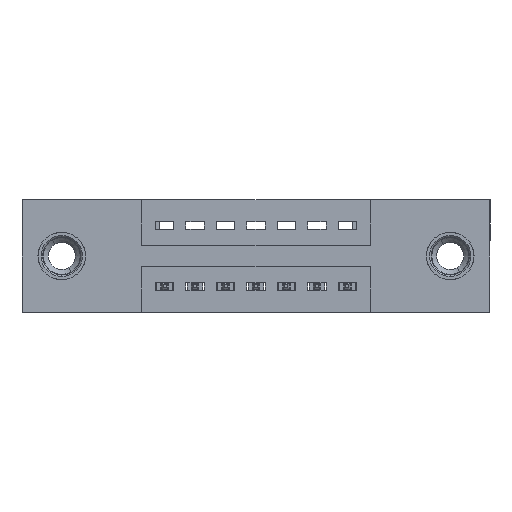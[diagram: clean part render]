
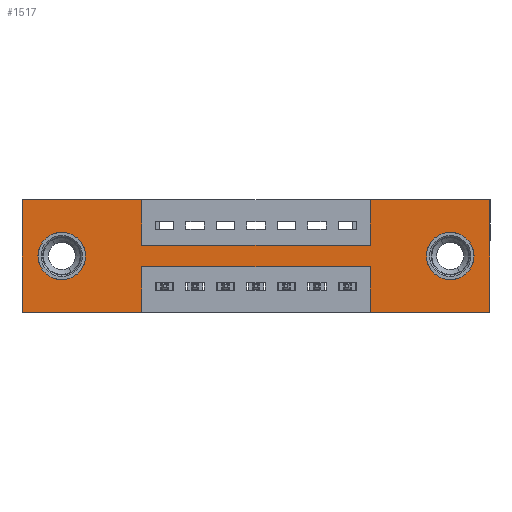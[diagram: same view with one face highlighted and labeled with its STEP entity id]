
A CAD part, front view. The second image highlights one B-rep face of the part: STEP entity #1517.
In plain terms, the highlighted planar face has unit normal (0, -1, 0).
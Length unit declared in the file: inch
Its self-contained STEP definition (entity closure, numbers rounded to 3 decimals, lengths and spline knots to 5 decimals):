
#113 = VERTEX_POINT ( 'NONE', #7295 ) ;
#277 = ORIENTED_EDGE ( 'NONE', *, *, #6809, .F. ) ;
#323 = VERTEX_POINT ( 'NONE', #5345 ) ;
#360 = CARTESIAN_POINT ( 'NONE',  ( 0.13, 0., -0.263 ) ) ;
#495 = EDGE_CURVE ( 'NONE', #4745, #14219, #9476, .T. ) ;
#669 = CARTESIAN_POINT ( 'NONE',  ( 1.405, 0., -0.185 ) ) ;
#693 = EDGE_CURVE ( 'NONE', #113, #14028, #1950, .T. ) ;
#728 = AXIS2_PLACEMENT_3D ( 'NONE', #6115, #1518, #10643 ) ;
#738 = ORIENTED_EDGE ( 'NONE', *, *, #2934, .F. ) ;
#791 = LINE ( 'NONE', #8367, #1706 ) ;
#948 = CARTESIAN_POINT ( 'NONE',  ( 1.535, 0., 0. ) ) ;
#960 = EDGE_CURVE ( 'NONE', #10817, #13637, #3906, .T. ) ;
#1022 = CARTESIAN_POINT ( 'NONE',  ( 0., 0., 0. ) ) ;
#1066 = CARTESIAN_POINT ( 'NONE',  ( 0.3925, 0., -0.37 ) ) ;
#1148 = DIRECTION ( 'NONE',  ( -1., 0., 0. ) ) ;
#1242 = ORIENTED_EDGE ( 'NONE', *, *, #4213, .F. ) ;
#1282 = AXIS2_PLACEMENT_3D ( 'NONE', #13565, #6637, #8975 ) ;
#1306 = ORIENTED_EDGE ( 'NONE', *, *, #960, .T. ) ;
#1517 = ADVANCED_FACE ( 'NONE', ( #7096, #2469, #4066 ), #3292, .T. ) ;
#1518 = DIRECTION ( 'NONE',  ( 0., 1., 0. ) ) ;
#1637 = ORIENTED_EDGE ( 'NONE', *, *, #8611, .F. ) ;
#1706 = VECTOR ( 'NONE', #1148, 39.37008 ) ;
#1950 = LINE ( 'NONE', #1022, #2303 ) ;
#1959 = CARTESIAN_POINT ( 'NONE',  ( 1.1425, 0., 0. ) ) ;
#1962 = CARTESIAN_POINT ( 'NONE',  ( 1.1425, 0., -0.15 ) ) ;
#2038 = AXIS2_PLACEMENT_3D ( 'NONE', #669, #14268, #8656 ) ;
#2050 = DIRECTION ( 'NONE',  ( 0., 0., 1. ) ) ;
#2103 = AXIS2_PLACEMENT_3D ( 'NONE', #7511, #5322, #13303 ) ;
#2284 = CARTESIAN_POINT ( 'NONE',  ( 0.3925, 0., 0. ) ) ;
#2303 = VECTOR ( 'NONE', #2050, 39.37008 ) ;
#2421 = VERTEX_POINT ( 'NONE', #4828 ) ;
#2469 = FACE_BOUND ( 'NONE', #14363, .T. ) ;
#2500 = ORIENTED_EDGE ( 'NONE', *, *, #9131, .F. ) ;
#2554 = DIRECTION ( 'NONE',  ( 0., 1., 0. ) ) ;
#2634 = CARTESIAN_POINT ( 'NONE',  ( 0.3925, 0., -0.22 ) ) ;
#2934 = EDGE_CURVE ( 'NONE', #9582, #8300, #12788, .T. ) ;
#2944 = LINE ( 'NONE', #948, #11658 ) ;
#3166 = DIRECTION ( 'NONE',  ( 0., 0., -1. ) ) ;
#3292 = PLANE ( 'NONE',  #1282 ) ;
#3645 = ORIENTED_EDGE ( 'NONE', *, *, #4347, .F. ) ;
#3849 = ORIENTED_EDGE ( 'NONE', *, *, #4507, .T. ) ;
#3906 = CIRCLE ( 'NONE', #8739, 0.078 ) ;
#4066 = FACE_OUTER_BOUND ( 'NONE', #9863, .T. ) ;
#4147 = DIRECTION ( 'NONE',  ( -1., 0., 0. ) ) ;
#4213 = EDGE_CURVE ( 'NONE', #11469, #14191, #9954, .T. ) ;
#4347 = EDGE_CURVE ( 'NONE', #14191, #113, #791, .T. ) ;
#4355 = ORIENTED_EDGE ( 'NONE', *, *, #5739, .F. ) ;
#4430 = CARTESIAN_POINT ( 'NONE',  ( 0., 0., 0. ) ) ;
#4507 = EDGE_CURVE ( 'NONE', #13637, #10817, #5997, .T. ) ;
#4537 = LINE ( 'NONE', #5249, #12949 ) ;
#4667 = ORIENTED_EDGE ( 'NONE', *, *, #693, .F. ) ;
#4745 = VERTEX_POINT ( 'NONE', #1959 ) ;
#4828 = CARTESIAN_POINT ( 'NONE',  ( 1.535, 0., -0.37 ) ) ;
#4985 = DIRECTION ( 'NONE',  ( 0., 0., 1. ) ) ;
#5249 = CARTESIAN_POINT ( 'NONE',  ( 0., 0., -0.37 ) ) ;
#5322 = DIRECTION ( 'NONE',  ( 0., 1., 0. ) ) ;
#5345 = CARTESIAN_POINT ( 'NONE',  ( 1.405, 0., -0.263 ) ) ;
#5379 = EDGE_CURVE ( 'NONE', #14385, #323, #12201, .T. ) ;
#5446 = EDGE_LOOP ( 'NONE', ( #7720, #6292 ) ) ;
#5739 = EDGE_CURVE ( 'NONE', #14219, #2421, #2944, .T. ) ;
#5985 = CARTESIAN_POINT ( 'NONE',  ( 1.405, 0., -0.107 ) ) ;
#5997 = CIRCLE ( 'NONE', #728, 0.078 ) ;
#6115 = CARTESIAN_POINT ( 'NONE',  ( 0.13, 0., -0.185 ) ) ;
#6256 = CARTESIAN_POINT ( 'NONE',  ( 1.1425, 0., -0.37 ) ) ;
#6292 = ORIENTED_EDGE ( 'NONE', *, *, #9628, .T. ) ;
#6389 = CIRCLE ( 'NONE', #2038, 0.078 ) ;
#6414 = DIRECTION ( 'NONE',  ( -1., 0., 0. ) ) ;
#6459 = EDGE_CURVE ( 'NONE', #14028, #9582, #10750, .T. ) ;
#6483 = VERTEX_POINT ( 'NONE', #7733 ) ;
#6513 = VERTEX_POINT ( 'NONE', #1962 ) ;
#6637 = DIRECTION ( 'NONE',  ( 0., -1., 0. ) ) ;
#6786 = VERTEX_POINT ( 'NONE', #8350 ) ;
#6809 = EDGE_CURVE ( 'NONE', #6513, #4745, #8425, .T. ) ;
#7096 = FACE_BOUND ( 'NONE', #5446, .T. ) ;
#7295 = CARTESIAN_POINT ( 'NONE',  ( 0., 0., -0.37 ) ) ;
#7365 = CARTESIAN_POINT ( 'NONE',  ( 0.3925, 0., 0. ) ) ;
#7488 = ORIENTED_EDGE ( 'NONE', *, *, #6459, .F. ) ;
#7511 = CARTESIAN_POINT ( 'NONE',  ( 1.405, 0., -0.185 ) ) ;
#7706 = VECTOR ( 'NONE', #11027, 39.37008 ) ;
#7720 = ORIENTED_EDGE ( 'NONE', *, *, #5379, .T. ) ;
#7733 = CARTESIAN_POINT ( 'NONE',  ( 1.1425, 0., -0.37 ) ) ;
#7863 = CARTESIAN_POINT ( 'NONE',  ( 0.3925, 0., -0.15 ) ) ;
#7884 = DIRECTION ( 'NONE',  ( 0., 0., -1. ) ) ;
#8300 = VERTEX_POINT ( 'NONE', #10331 ) ;
#8350 = CARTESIAN_POINT ( 'NONE',  ( 1.1425, 0., -0.22 ) ) ;
#8367 = CARTESIAN_POINT ( 'NONE',  ( 0., 0., -0.37 ) ) ;
#8425 = LINE ( 'NONE', #10886, #9696 ) ;
#8579 = DIRECTION ( 'NONE',  ( 0., 0., 1. ) ) ;
#8611 = EDGE_CURVE ( 'NONE', #8300, #6513, #11574, .T. ) ;
#8656 = DIRECTION ( 'NONE',  ( 0., 0., -1. ) ) ;
#8739 = AXIS2_PLACEMENT_3D ( 'NONE', #10676, #2554, #4985 ) ;
#8975 = DIRECTION ( 'NONE',  ( 0., 0., -1. ) ) ;
#9131 = EDGE_CURVE ( 'NONE', #6786, #11469, #10685, .T. ) ;
#9382 = VECTOR ( 'NONE', #8579, 39.37008 ) ;
#9476 = LINE ( 'NONE', #4430, #13935 ) ;
#9582 = VERTEX_POINT ( 'NONE', #7365 ) ;
#9628 = EDGE_CURVE ( 'NONE', #323, #14385, #6389, .T. ) ;
#9696 = VECTOR ( 'NONE', #14321, 39.37008 ) ;
#9863 = EDGE_LOOP ( 'NONE', ( #1242, #2500, #14720, #12967, #4355, #14806, #277, #1637, #738, #7488, #4667, #3645 ) ) ;
#9954 = LINE ( 'NONE', #12232, #11730 ) ;
#9975 = CARTESIAN_POINT ( 'NONE',  ( 0., 0., 0. ) ) ;
#10151 = VECTOR ( 'NONE', #6414, 39.37008 ) ;
#10331 = CARTESIAN_POINT ( 'NONE',  ( 0.3925, 0., -0.15 ) ) ;
#10643 = DIRECTION ( 'NONE',  ( 0., 0., 1. ) ) ;
#10676 = CARTESIAN_POINT ( 'NONE',  ( 0.13, 0., -0.185 ) ) ;
#10685 = LINE ( 'NONE', #12040, #10151 ) ;
#10750 = LINE ( 'NONE', #14410, #7706 ) ;
#10817 = VERTEX_POINT ( 'NONE', #360 ) ;
#10886 = CARTESIAN_POINT ( 'NONE',  ( 1.1425, 0., 0. ) ) ;
#11027 = DIRECTION ( 'NONE',  ( 1., 0., 0. ) ) ;
#11203 = DIRECTION ( 'NONE',  ( 1., 0., 0. ) ) ;
#11445 = DIRECTION ( 'NONE',  ( 0., 0., -1. ) ) ;
#11446 = CARTESIAN_POINT ( 'NONE',  ( 1.535, 0., 0. ) ) ;
#11469 = VERTEX_POINT ( 'NONE', #2634 ) ;
#11493 = LINE ( 'NONE', #6256, #9382 ) ;
#11533 = VECTOR ( 'NONE', #11445, 39.37008 ) ;
#11574 = LINE ( 'NONE', #7863, #14471 ) ;
#11658 = VECTOR ( 'NONE', #7884, 39.37008 ) ;
#11730 = VECTOR ( 'NONE', #3166, 39.37008 ) ;
#12040 = CARTESIAN_POINT ( 'NONE',  ( 0.3925, 0., -0.22 ) ) ;
#12201 = CIRCLE ( 'NONE', #2103, 0.078 ) ;
#12232 = CARTESIAN_POINT ( 'NONE',  ( 0.3925, 0., -0.37 ) ) ;
#12453 = DIRECTION ( 'NONE',  ( 1., 0., 0. ) ) ;
#12788 = LINE ( 'NONE', #2284, #11533 ) ;
#12949 = VECTOR ( 'NONE', #4147, 39.37008 ) ;
#12967 = ORIENTED_EDGE ( 'NONE', *, *, #13505, .F. ) ;
#13303 = DIRECTION ( 'NONE',  ( 0., 0., -1. ) ) ;
#13505 = EDGE_CURVE ( 'NONE', #2421, #6483, #4537, .T. ) ;
#13565 = CARTESIAN_POINT ( 'NONE',  ( 0., 0., -0.37 ) ) ;
#13637 = VERTEX_POINT ( 'NONE', #14686 ) ;
#13911 = EDGE_CURVE ( 'NONE', #6483, #6786, #11493, .T. ) ;
#13935 = VECTOR ( 'NONE', #11203, 39.37008 ) ;
#14028 = VERTEX_POINT ( 'NONE', #9975 ) ;
#14191 = VERTEX_POINT ( 'NONE', #1066 ) ;
#14219 = VERTEX_POINT ( 'NONE', #11446 ) ;
#14268 = DIRECTION ( 'NONE',  ( 0., 1., 0. ) ) ;
#14321 = DIRECTION ( 'NONE',  ( 0., 0., 1. ) ) ;
#14363 = EDGE_LOOP ( 'NONE', ( #3849, #1306 ) ) ;
#14385 = VERTEX_POINT ( 'NONE', #5985 ) ;
#14410 = CARTESIAN_POINT ( 'NONE',  ( 0., 0., 0. ) ) ;
#14471 = VECTOR ( 'NONE', #12453, 39.37008 ) ;
#14686 = CARTESIAN_POINT ( 'NONE',  ( 0.13, 0., -0.107 ) ) ;
#14720 = ORIENTED_EDGE ( 'NONE', *, *, #13911, .F. ) ;
#14806 = ORIENTED_EDGE ( 'NONE', *, *, #495, .F. ) ;
